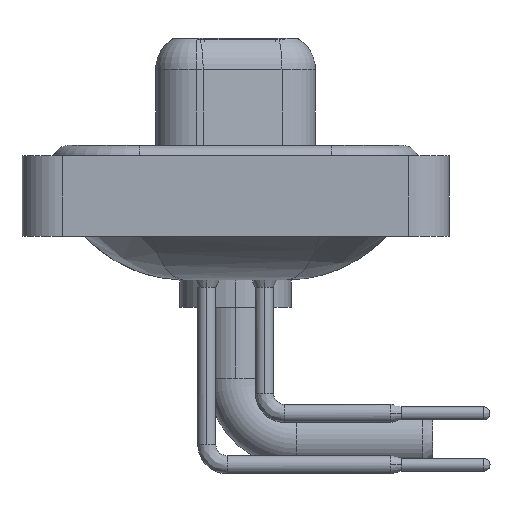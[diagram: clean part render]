
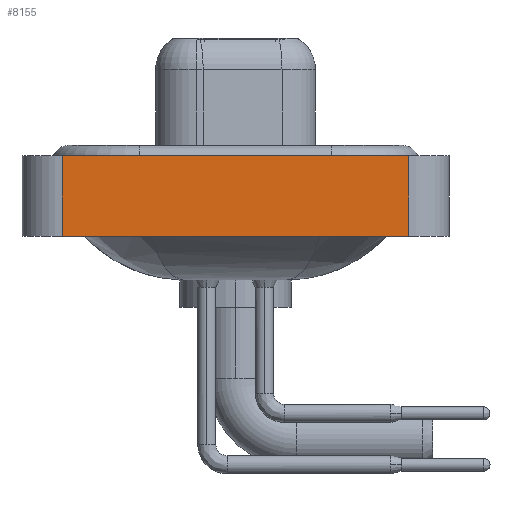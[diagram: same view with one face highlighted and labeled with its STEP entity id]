
A CAD part, left-side view. The second image highlights one B-rep face of the part: STEP entity #8155.
In plain terms, the highlighted planar face has unit normal (-1, 0, 0).
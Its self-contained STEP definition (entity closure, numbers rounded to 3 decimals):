
#159 = EDGE_CURVE ( 'NONE', #8963, #17443, #13223, .T. ) ;
#825 = CARTESIAN_POINT ( 'NONE',  ( -7.25, -8.55, -3.6 ) ) ;
#3021 = LINE ( 'NONE', #6040, #10856 ) ;
#3738 = CARTESIAN_POINT ( 'NONE',  ( -7.25, -8.55, -3.6 ) ) ;
#4003 = DIRECTION ( 'NONE',  ( 0., 0., 1. ) ) ;
#4029 = DIRECTION ( 'NONE',  ( 0., 0., 1. ) ) ;
#5163 = CARTESIAN_POINT ( 'NONE',  ( -7.25, 8.55, -3.6 ) ) ;
#6040 = CARTESIAN_POINT ( 'NONE',  ( -7.25, -8.55, -3.6 ) ) ;
#6304 = CARTESIAN_POINT ( 'NONE',  ( -7.25, 8.55, 0.4 ) ) ;
#6362 = ORIENTED_EDGE ( 'NONE', *, *, #9783, .T. ) ;
#6890 = EDGE_CURVE ( 'NONE', #16379, #9512, #11460, .T. ) ;
#6910 = LINE ( 'NONE', #14615, #10197 ) ;
#6933 = DIRECTION ( 'NONE',  ( 0., -1., 0. ) ) ;
#7161 = ORIENTED_EDGE ( 'NONE', *, *, #8626, .F. ) ;
#7893 = ORIENTED_EDGE ( 'NONE', *, *, #159, .F. ) ;
#8155 = ADVANCED_FACE ( 'NONE', ( #17549 ), #8560, .T. ) ;
#8560 = PLANE ( 'NONE',  #11770 ) ;
#8626 = EDGE_CURVE ( 'NONE', #16379, #8963, #6910, .T. ) ;
#8840 = DIRECTION ( 'NONE',  ( 0., -1., 0. ) ) ;
#8963 = VERTEX_POINT ( 'NONE', #6304 ) ;
#9512 = VERTEX_POINT ( 'NONE', #3738 ) ;
#9689 = VECTOR ( 'NONE', #8840, 1000. ) ;
#9783 = EDGE_CURVE ( 'NONE', #9512, #17443, #3021, .T. ) ;
#10197 = VECTOR ( 'NONE', #4003, 1000. ) ;
#10239 = CARTESIAN_POINT ( 'NONE',  ( -7.25, -8.55, 0.4 ) ) ;
#10856 = VECTOR ( 'NONE', #15036, 1000. ) ;
#10884 = ORIENTED_EDGE ( 'NONE', *, *, #6890, .T. ) ;
#11460 = LINE ( 'NONE', #17548, #14027 ) ;
#11770 = AXIS2_PLACEMENT_3D ( 'NONE', #825, #16434, #4029 ) ;
#13223 = LINE ( 'NONE', #10239, #9689 ) ;
#14027 = VECTOR ( 'NONE', #6933, 1000. ) ;
#14615 = CARTESIAN_POINT ( 'NONE',  ( -7.25, 8.55, -3.6 ) ) ;
#15036 = DIRECTION ( 'NONE',  ( 0., 0., 1. ) ) ;
#15809 = CARTESIAN_POINT ( 'NONE',  ( -7.25, -8.55, 0.4 ) ) ;
#16379 = VERTEX_POINT ( 'NONE', #5163 ) ;
#16434 = DIRECTION ( 'NONE',  ( -1., 0., 0. ) ) ;
#17443 = VERTEX_POINT ( 'NONE', #15809 ) ;
#17548 = CARTESIAN_POINT ( 'NONE',  ( -7.25, -8.55, -3.6 ) ) ;
#17549 = FACE_OUTER_BOUND ( 'NONE', #19455, .T. ) ;
#19455 = EDGE_LOOP ( 'NONE', ( #6362, #7893, #7161, #10884 ) ) ;
